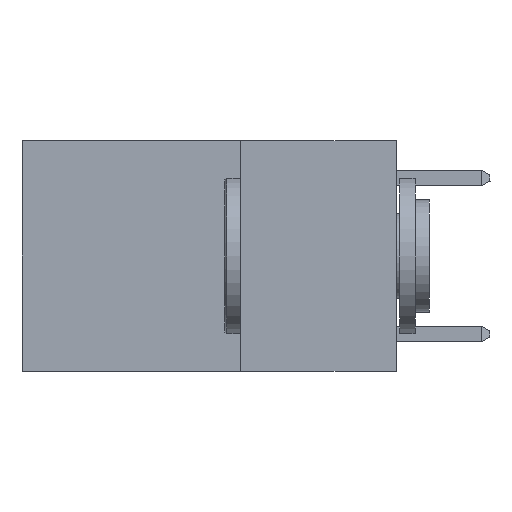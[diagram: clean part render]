
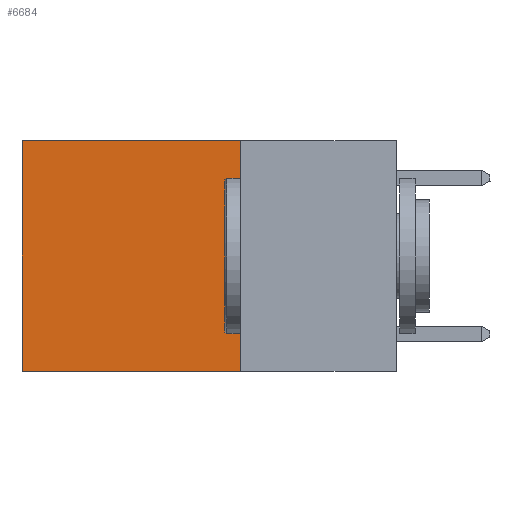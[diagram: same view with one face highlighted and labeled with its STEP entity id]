
A CAD part, left-side view. The second image highlights one B-rep face of the part: STEP entity #6684.
In plain terms, the highlighted planar face has unit normal (-1, 0, 0).
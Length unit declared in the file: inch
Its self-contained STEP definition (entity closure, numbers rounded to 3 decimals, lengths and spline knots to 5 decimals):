
#657 = EDGE_CURVE ( 'NONE', #12256, #12116, #7515, .T. ) ;
#1410 = EDGE_CURVE ( 'NONE', #11681, #12116, #10200, .T. ) ;
#1933 = DIRECTION ( 'NONE',  ( 0., 0., -1. ) ) ;
#2267 = CARTESIAN_POINT ( 'NONE',  ( 0.2625, 0.6, 0. ) ) ;
#2865 = CARTESIAN_POINT ( 'NONE',  ( 0.2625, 0.25, -0.37 ) ) ;
#3190 = LINE ( 'NONE', #7427, #13534 ) ;
#3390 = CARTESIAN_POINT ( 'NONE',  ( 0.2625, 0.25, 0. ) ) ;
#3991 = PLANE ( 'NONE',  #8718 ) ;
#4640 = EDGE_CURVE ( 'NONE', #8125, #11681, #10536, .T. ) ;
#5238 = DIRECTION ( 'NONE',  ( 1., 0., 0. ) ) ;
#5759 = CARTESIAN_POINT ( 'NONE',  ( 0.2625, 0.25, 0. ) ) ;
#6684 = ADVANCED_FACE ( 'NONE', ( #6756 ), #3991, .F. ) ;
#6756 = FACE_OUTER_BOUND ( 'NONE', #9225, .T. ) ;
#7011 = ORIENTED_EDGE ( 'NONE', *, *, #657, .F. ) ;
#7427 = CARTESIAN_POINT ( 'NONE',  ( 0.2625, 0.25, 0. ) ) ;
#7515 = LINE ( 'NONE', #10336, #8179 ) ;
#8125 = VERTEX_POINT ( 'NONE', #3390 ) ;
#8179 = VECTOR ( 'NONE', #12442, 39.37008 ) ;
#8473 = VECTOR ( 'NONE', #9756, 39.37008 ) ;
#8718 = AXIS2_PLACEMENT_3D ( 'NONE', #9550, #5238, #12614 ) ;
#9225 = EDGE_LOOP ( 'NONE', ( #9618, #7011, #12490, #9580 ) ) ;
#9550 = CARTESIAN_POINT ( 'NONE',  ( 0.2625, 0.25, 0. ) ) ;
#9580 = ORIENTED_EDGE ( 'NONE', *, *, #4640, .T. ) ;
#9618 = ORIENTED_EDGE ( 'NONE', *, *, #1410, .T. ) ;
#9756 = DIRECTION ( 'NONE',  ( 0., 0., -1. ) ) ;
#10200 = LINE ( 'NONE', #2267, #8473 ) ;
#10336 = CARTESIAN_POINT ( 'NONE',  ( 0.2625, 0.25, -0.37 ) ) ;
#10536 = LINE ( 'NONE', #5759, #11678 ) ;
#10624 = CARTESIAN_POINT ( 'NONE',  ( 0.2625, 0.6, 0. ) ) ;
#11194 = DIRECTION ( 'NONE',  ( 0., 1., 0. ) ) ;
#11678 = VECTOR ( 'NONE', #11194, 39.37008 ) ;
#11681 = VERTEX_POINT ( 'NONE', #10624 ) ;
#12116 = VERTEX_POINT ( 'NONE', #12540 ) ;
#12256 = VERTEX_POINT ( 'NONE', #2865 ) ;
#12442 = DIRECTION ( 'NONE',  ( 0., 1., 0. ) ) ;
#12490 = ORIENTED_EDGE ( 'NONE', *, *, #13795, .F. ) ;
#12540 = CARTESIAN_POINT ( 'NONE',  ( 0.2625, 0.6, -0.37 ) ) ;
#12614 = DIRECTION ( 'NONE',  ( 0., 0., -1. ) ) ;
#13534 = VECTOR ( 'NONE', #1933, 39.37008 ) ;
#13795 = EDGE_CURVE ( 'NONE', #8125, #12256, #3190, .T. ) ;
